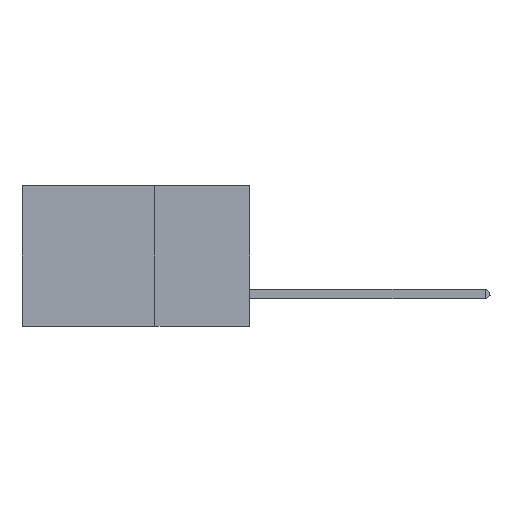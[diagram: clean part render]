
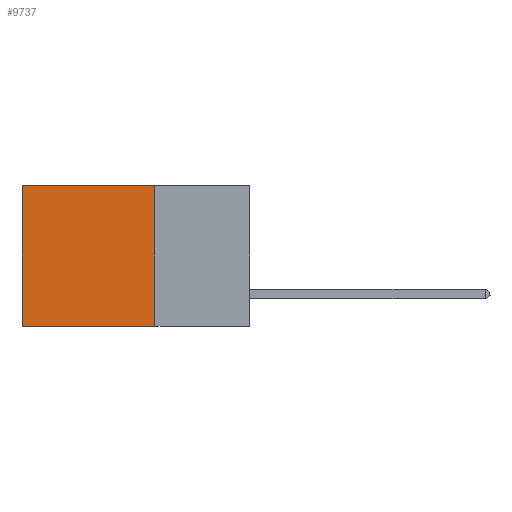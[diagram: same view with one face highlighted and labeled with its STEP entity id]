
A CAD part, left-side view. The second image highlights one B-rep face of the part: STEP entity #9737.
In plain terms, the highlighted planar face has unit normal (-1, 0, 0).
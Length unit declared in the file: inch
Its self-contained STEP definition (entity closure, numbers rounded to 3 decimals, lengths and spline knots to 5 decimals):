
#1993 = PLANE ( 'NONE',  #10935 ) ;
#2160 = VECTOR ( 'NONE', #14604, 39.37008 ) ;
#2294 = DIRECTION ( 'NONE',  ( 0., 1., 0. ) ) ;
#2516 = ORIENTED_EDGE ( 'NONE', *, *, #14123, .T. ) ;
#2859 = LINE ( 'NONE', #7085, #18693 ) ;
#2950 = VERTEX_POINT ( 'NONE', #3948 ) ;
#3162 = CARTESIAN_POINT ( 'NONE',  ( 0.2875, 0.25, -0.37 ) ) ;
#3508 = VERTEX_POINT ( 'NONE', #15355 ) ;
#3656 = EDGE_CURVE ( 'NONE', #14766, #12942, #19113, .T. ) ;
#3948 = CARTESIAN_POINT ( 'NONE',  ( 0.2875, 0.6, 0. ) ) ;
#4169 = CARTESIAN_POINT ( 'NONE',  ( 0.2875, 0.6, -0.37 ) ) ;
#5408 = DIRECTION ( 'NONE',  ( 0., 0., -1. ) ) ;
#6270 = LINE ( 'NONE', #17685, #2160 ) ;
#6376 = VECTOR ( 'NONE', #19744, 39.37008 ) ;
#7085 = CARTESIAN_POINT ( 'NONE',  ( 0.2875, 0.6, 0. ) ) ;
#7118 = DIRECTION ( 'NONE',  ( 1., 0., 0. ) ) ;
#8112 = EDGE_CURVE ( 'NONE', #2950, #12942, #2859, .T. ) ;
#9153 = LINE ( 'NONE', #14743, #11030 ) ;
#9737 = ADVANCED_FACE ( 'NONE', ( #16062 ), #1993, .F. ) ;
#10935 = AXIS2_PLACEMENT_3D ( 'NONE', #14309, #7118, #5408 ) ;
#11030 = VECTOR ( 'NONE', #2294, 39.37008 ) ;
#11048 = ORIENTED_EDGE ( 'NONE', *, *, #3656, .F. ) ;
#12862 = ORIENTED_EDGE ( 'NONE', *, *, #8112, .T. ) ;
#12942 = VERTEX_POINT ( 'NONE', #4169 ) ;
#13001 = ORIENTED_EDGE ( 'NONE', *, *, #14117, .F. ) ;
#14117 = EDGE_CURVE ( 'NONE', #3508, #14766, #6270, .T. ) ;
#14123 = EDGE_CURVE ( 'NONE', #3508, #2950, #9153, .T. ) ;
#14309 = CARTESIAN_POINT ( 'NONE',  ( 0.2875, 0.25, 0. ) ) ;
#14604 = DIRECTION ( 'NONE',  ( 0., 0., -1. ) ) ;
#14743 = CARTESIAN_POINT ( 'NONE',  ( 0.2875, 0.25, 0. ) ) ;
#14766 = VERTEX_POINT ( 'NONE', #3162 ) ;
#15261 = EDGE_LOOP ( 'NONE', ( #12862, #11048, #13001, #2516 ) ) ;
#15355 = CARTESIAN_POINT ( 'NONE',  ( 0.2875, 0.25, 0. ) ) ;
#16062 = FACE_OUTER_BOUND ( 'NONE', #15261, .T. ) ;
#16689 = CARTESIAN_POINT ( 'NONE',  ( 0.2875, 0.25, -0.37 ) ) ;
#17685 = CARTESIAN_POINT ( 'NONE',  ( 0.2875, 0.25, 0. ) ) ;
#18009 = DIRECTION ( 'NONE',  ( 0., 0., -1. ) ) ;
#18693 = VECTOR ( 'NONE', #18009, 39.37008 ) ;
#19113 = LINE ( 'NONE', #16689, #6376 ) ;
#19744 = DIRECTION ( 'NONE',  ( 0., 1., 0. ) ) ;
